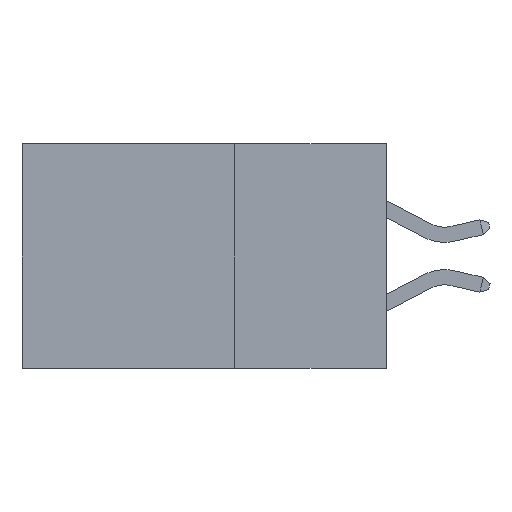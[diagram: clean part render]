
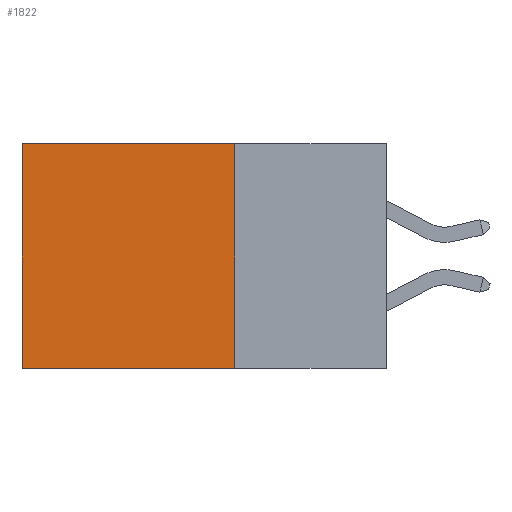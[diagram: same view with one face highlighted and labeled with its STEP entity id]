
A CAD part, left-side view. The second image highlights one B-rep face of the part: STEP entity #1822.
In plain terms, the highlighted planar face has unit normal (-1, 0, 0).
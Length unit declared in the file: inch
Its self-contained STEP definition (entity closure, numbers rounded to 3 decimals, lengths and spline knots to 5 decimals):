
#744 = DIRECTION ( 'NONE',  ( 0., 1., 0. ) ) ;
#764 = CARTESIAN_POINT ( 'NONE',  ( 0.2615, 0.25, 0. ) ) ;
#913 = VERTEX_POINT ( 'NONE', #14994 ) ;
#969 = VECTOR ( 'NONE', #7313, 39.37008 ) ;
#1124 = LINE ( 'NONE', #764, #14666 ) ;
#1581 = CARTESIAN_POINT ( 'NONE',  ( 0.2615, 0.25, -0.37 ) ) ;
#1822 = ADVANCED_FACE ( 'NONE', ( #13118 ), #15209, .F. ) ;
#2408 = VERTEX_POINT ( 'NONE', #8911 ) ;
#2548 = ORIENTED_EDGE ( 'NONE', *, *, #5079, .T. ) ;
#2872 = DIRECTION ( 'NONE',  ( 0., 1., 0. ) ) ;
#4012 = LINE ( 'NONE', #6296, #14335 ) ;
#4376 = VERTEX_POINT ( 'NONE', #5926 ) ;
#5079 = EDGE_CURVE ( 'NONE', #16205, #4376, #1124, .T. ) ;
#5926 = CARTESIAN_POINT ( 'NONE',  ( 0.2615, 0.6, 0. ) ) ;
#6296 = CARTESIAN_POINT ( 'NONE',  ( 0.2615, 0.25, -0.37 ) ) ;
#6513 = AXIS2_PLACEMENT_3D ( 'NONE', #10694, #12934, #12864 ) ;
#7313 = DIRECTION ( 'NONE',  ( 0., 0., -1. ) ) ;
#8325 = DIRECTION ( 'NONE',  ( 0., 0., -1. ) ) ;
#8624 = VECTOR ( 'NONE', #8325, 39.37008 ) ;
#8911 = CARTESIAN_POINT ( 'NONE',  ( 0.2615, 0.25, -0.37 ) ) ;
#9167 = EDGE_CURVE ( 'NONE', #2408, #913, #4012, .T. ) ;
#9824 = EDGE_CURVE ( 'NONE', #4376, #913, #11389, .T. ) ;
#10481 = ORIENTED_EDGE ( 'NONE', *, *, #9167, .F. ) ;
#10694 = CARTESIAN_POINT ( 'NONE',  ( 0.2615, 0.25, -0.37 ) ) ;
#11070 = EDGE_CURVE ( 'NONE', #16205, #2408, #16143, .T. ) ;
#11298 = EDGE_LOOP ( 'NONE', ( #13210, #10481, #16829, #2548 ) ) ;
#11389 = LINE ( 'NONE', #15317, #969 ) ;
#12864 = DIRECTION ( 'NONE',  ( 0., 0., -1. ) ) ;
#12934 = DIRECTION ( 'NONE',  ( 1., 0., 0. ) ) ;
#13118 = FACE_OUTER_BOUND ( 'NONE', #11298, .T. ) ;
#13210 = ORIENTED_EDGE ( 'NONE', *, *, #9824, .T. ) ;
#14335 = VECTOR ( 'NONE', #2872, 39.37008 ) ;
#14666 = VECTOR ( 'NONE', #744, 39.37008 ) ;
#14994 = CARTESIAN_POINT ( 'NONE',  ( 0.2615, 0.6, -0.37 ) ) ;
#15209 = PLANE ( 'NONE',  #6513 ) ;
#15317 = CARTESIAN_POINT ( 'NONE',  ( 0.2615, 0.6, -0.37 ) ) ;
#16143 = LINE ( 'NONE', #1581, #8624 ) ;
#16205 = VERTEX_POINT ( 'NONE', #17256 ) ;
#16829 = ORIENTED_EDGE ( 'NONE', *, *, #11070, .F. ) ;
#17256 = CARTESIAN_POINT ( 'NONE',  ( 0.2615, 0.25, 0. ) ) ;
